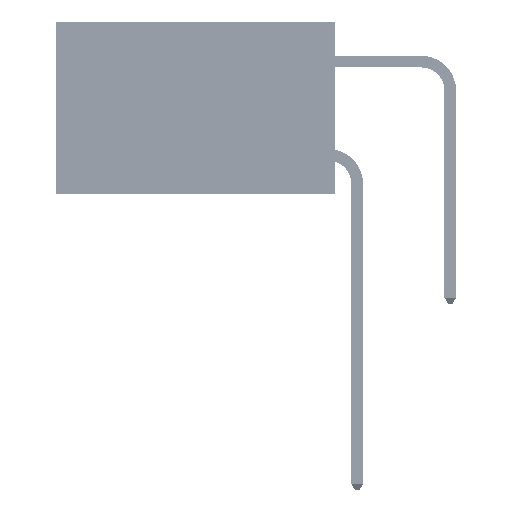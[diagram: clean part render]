
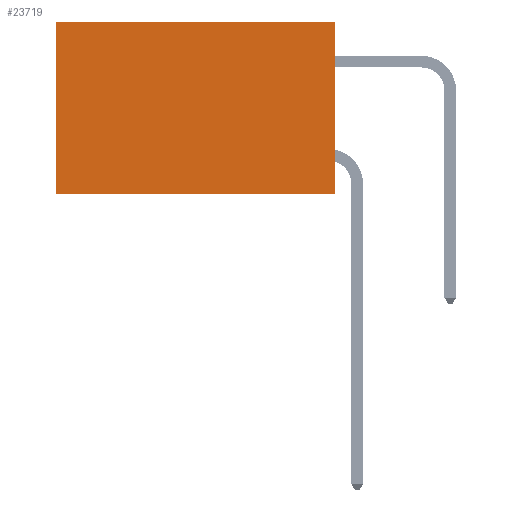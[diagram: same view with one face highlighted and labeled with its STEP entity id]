
A CAD part, left-side view. The second image highlights one B-rep face of the part: STEP entity #23719.
In plain terms, the highlighted planar face has unit normal (-1, 0, 0).
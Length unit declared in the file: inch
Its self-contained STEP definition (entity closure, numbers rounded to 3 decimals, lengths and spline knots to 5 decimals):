
#1093 = ORIENTED_EDGE ( 'NONE', *, *, #36867, .F. ) ;
#1328 = CARTESIAN_POINT ( 'NONE',  ( 0.2875, 0., -0.37 ) ) ;
#4240 = VECTOR ( 'NONE', #20332, 39.37008 ) ;
#4868 = EDGE_CURVE ( 'NONE', #17310, #7144, #31101, .T. ) ;
#5018 = CARTESIAN_POINT ( 'NONE',  ( 0.2875, 0., -0.37 ) ) ;
#5277 = CARTESIAN_POINT ( 'NONE',  ( 0.2875, 0.6, -0.37 ) ) ;
#7022 = DIRECTION ( 'NONE',  ( 0., 0., -1. ) ) ;
#7144 = VERTEX_POINT ( 'NONE', #1328 ) ;
#7471 = CARTESIAN_POINT ( 'NONE',  ( 0.2875, 0., 0. ) ) ;
#9233 = CARTESIAN_POINT ( 'NONE',  ( 0.2875, 0., 0. ) ) ;
#11850 = EDGE_LOOP ( 'NONE', ( #30501, #1093, #49193, #45880 ) ) ;
#13314 = VECTOR ( 'NONE', #13808, 39.37008 ) ;
#13808 = DIRECTION ( 'NONE',  ( 0., 0., -1. ) ) ;
#14000 = FACE_OUTER_BOUND ( 'NONE', #11850, .T. ) ;
#15122 = DIRECTION ( 'NONE',  ( 0., 0., -1. ) ) ;
#15179 = CARTESIAN_POINT ( 'NONE',  ( 0.2875, 0.6, 0. ) ) ;
#15459 = DIRECTION ( 'NONE',  ( 1., 0., 0. ) ) ;
#16801 = CARTESIAN_POINT ( 'NONE',  ( 0.2875, 0., 0. ) ) ;
#17310 = VERTEX_POINT ( 'NONE', #16801 ) ;
#20332 = DIRECTION ( 'NONE',  ( 0., 1., 0. ) ) ;
#21129 = DIRECTION ( 'NONE',  ( 0., 1., 0. ) ) ;
#22956 = VECTOR ( 'NONE', #7022, 39.37008 ) ;
#22995 = VERTEX_POINT ( 'NONE', #15179 ) ;
#23427 = EDGE_CURVE ( 'NONE', #17310, #22995, #45275, .T. ) ;
#23719 = ADVANCED_FACE ( 'NONE', ( #14000 ), #38608, .F. ) ;
#25029 = EDGE_CURVE ( 'NONE', #22995, #31714, #38345, .T. ) ;
#26474 = CARTESIAN_POINT ( 'NONE',  ( 0.2875, 0.6, 0. ) ) ;
#28741 = LINE ( 'NONE', #5018, #4240 ) ;
#29076 = CARTESIAN_POINT ( 'NONE',  ( 0.2875, 0., 0. ) ) ;
#30501 = ORIENTED_EDGE ( 'NONE', *, *, #25029, .T. ) ;
#31101 = LINE ( 'NONE', #9233, #13314 ) ;
#31714 = VERTEX_POINT ( 'NONE', #5277 ) ;
#35463 = VECTOR ( 'NONE', #21129, 39.37008 ) ;
#36867 = EDGE_CURVE ( 'NONE', #7144, #31714, #28741, .T. ) ;
#38345 = LINE ( 'NONE', #26474, #22956 ) ;
#38509 = AXIS2_PLACEMENT_3D ( 'NONE', #7471, #15459, #15122 ) ;
#38608 = PLANE ( 'NONE',  #38509 ) ;
#45275 = LINE ( 'NONE', #29076, #35463 ) ;
#45880 = ORIENTED_EDGE ( 'NONE', *, *, #23427, .T. ) ;
#49193 = ORIENTED_EDGE ( 'NONE', *, *, #4868, .F. ) ;
